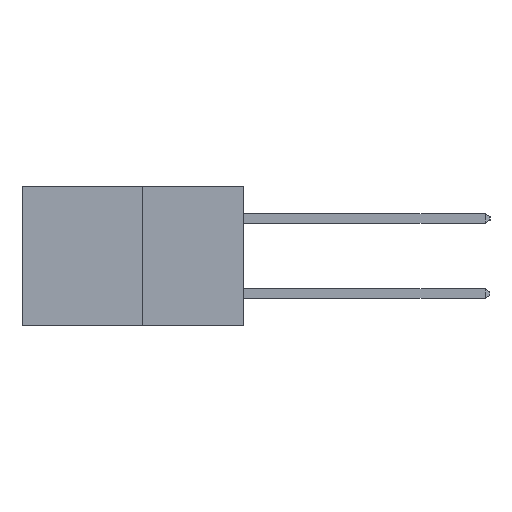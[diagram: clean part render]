
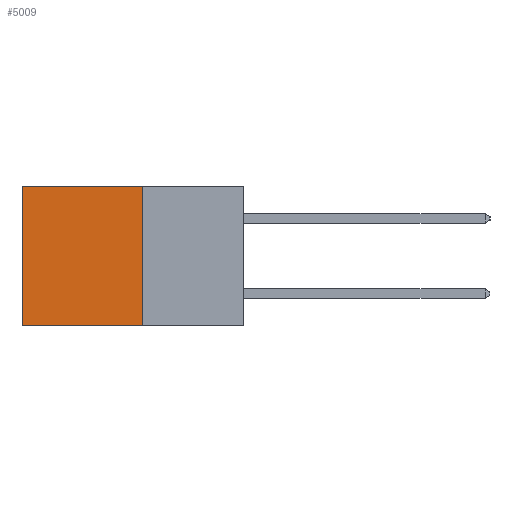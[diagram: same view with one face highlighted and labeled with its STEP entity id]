
A CAD part, left-side view. The second image highlights one B-rep face of the part: STEP entity #5009.
In plain terms, the highlighted planar face has unit normal (-1, 0, 0).
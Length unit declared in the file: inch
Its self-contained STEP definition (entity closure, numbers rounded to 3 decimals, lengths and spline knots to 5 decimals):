
#404 = AXIS2_PLACEMENT_3D ( 'NONE', #7202, #7159, #7157 ) ;
#437 = VERTEX_POINT ( 'NONE', #9018 ) ;
#444 = LINE ( 'NONE', #9452, #4253 ) ;
#462 = CARTESIAN_POINT ( 'NONE',  ( 0.277, 0.27, 0. ) ) ;
#1036 = CARTESIAN_POINT ( 'NONE',  ( 0.277, 0.27, -0.37 ) ) ;
#1810 = VERTEX_POINT ( 'NONE', #8851 ) ;
#1879 = VECTOR ( 'NONE', #5294, 39.37008 ) ;
#2096 = EDGE_CURVE ( 'NONE', #6221, #437, #2377, .T. ) ;
#2377 = LINE ( 'NONE', #4497, #4741 ) ;
#3524 = ORIENTED_EDGE ( 'NONE', *, *, #10773, .T. ) ;
#3554 = VECTOR ( 'NONE', #9040, 39.37008 ) ;
#4253 = VECTOR ( 'NONE', #10289, 39.37008 ) ;
#4497 = CARTESIAN_POINT ( 'NONE',  ( 0.277, 0.27, 0. ) ) ;
#4516 = LINE ( 'NONE', #5350, #1879 ) ;
#4592 = DIRECTION ( 'NONE',  ( 0., 1., 0. ) ) ;
#4741 = VECTOR ( 'NONE', #4592, 39.37008 ) ;
#4820 = EDGE_LOOP ( 'NONE', ( #3524, #8156, #9086, #7529 ) ) ;
#5009 = ADVANCED_FACE ( 'NONE', ( #5618 ), #7243, .F. ) ;
#5294 = DIRECTION ( 'NONE',  ( 0., 1., 0. ) ) ;
#5350 = CARTESIAN_POINT ( 'NONE',  ( 0.277, 0.27, -0.37 ) ) ;
#5618 = FACE_OUTER_BOUND ( 'NONE', #4820, .T. ) ;
#5875 = LINE ( 'NONE', #9614, #3554 ) ;
#6074 = VERTEX_POINT ( 'NONE', #1036 ) ;
#6221 = VERTEX_POINT ( 'NONE', #462 ) ;
#6446 = EDGE_CURVE ( 'NONE', #6221, #6074, #5875, .T. ) ;
#6592 = EDGE_CURVE ( 'NONE', #6074, #1810, #4516, .T. ) ;
#7157 = DIRECTION ( 'NONE',  ( 0., 0., -1. ) ) ;
#7159 = DIRECTION ( 'NONE',  ( 1., 0., 0. ) ) ;
#7202 = CARTESIAN_POINT ( 'NONE',  ( 0.277, 0.27, -0.37 ) ) ;
#7243 = PLANE ( 'NONE',  #404 ) ;
#7529 = ORIENTED_EDGE ( 'NONE', *, *, #2096, .T. ) ;
#8156 = ORIENTED_EDGE ( 'NONE', *, *, #6592, .F. ) ;
#8851 = CARTESIAN_POINT ( 'NONE',  ( 0.277, 0.59, -0.37 ) ) ;
#9018 = CARTESIAN_POINT ( 'NONE',  ( 0.277, 0.59, 0. ) ) ;
#9040 = DIRECTION ( 'NONE',  ( 0., 0., -1. ) ) ;
#9086 = ORIENTED_EDGE ( 'NONE', *, *, #6446, .F. ) ;
#9452 = CARTESIAN_POINT ( 'NONE',  ( 0.277, 0.59, -0.37 ) ) ;
#9614 = CARTESIAN_POINT ( 'NONE',  ( 0.277, 0.27, -0.37 ) ) ;
#10289 = DIRECTION ( 'NONE',  ( 0., 0., -1. ) ) ;
#10773 = EDGE_CURVE ( 'NONE', #437, #1810, #444, .T. ) ;
